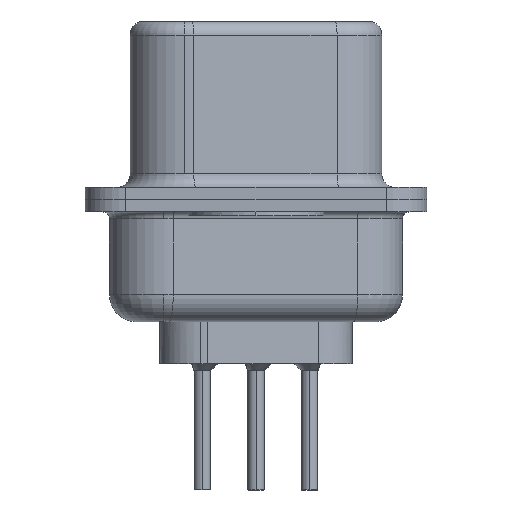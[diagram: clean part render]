
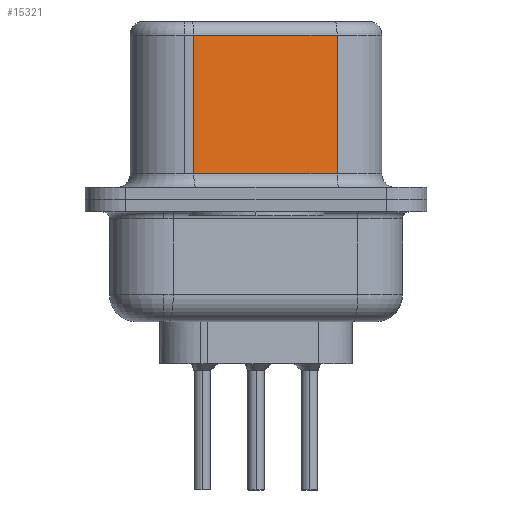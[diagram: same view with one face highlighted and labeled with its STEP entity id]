
A CAD part, left-side view. The second image highlights one B-rep face of the part: STEP entity #15321.
In plain terms, the highlighted planar face has unit normal (-0.985, -0.174, 0).
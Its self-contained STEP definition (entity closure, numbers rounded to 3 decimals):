
#120 = VECTOR ( 'NONE', #17267, 1000. ) ;
#445 = VECTOR ( 'NONE', #6712, 1000. ) ;
#1651 = FACE_OUTER_BOUND ( 'NONE', #18464, .T. ) ;
#1810 = ORIENTED_EDGE ( 'NONE', *, *, #16075, .T. ) ;
#2435 = DIRECTION ( 'NONE',  ( -0.174, 0.985, 0. ) ) ;
#2598 = ORIENTED_EDGE ( 'NONE', *, *, #7404, .T. ) ;
#3261 = CARTESIAN_POINT ( 'NONE',  ( 4.546, -2.987, 0.95 ) ) ;
#3389 = CARTESIAN_POINT ( 'NONE',  ( 4.546, -2.987, 6.07 ) ) ;
#5080 = CARTESIAN_POINT ( 'NONE',  ( 4.546, -2.987, 0.95 ) ) ;
#5292 = CARTESIAN_POINT ( 'NONE',  ( 3.615, 2.293, 6.57 ) ) ;
#5322 = DIRECTION ( 'NONE',  ( 0.985, 0.174, 0. ) ) ;
#6712 = DIRECTION ( 'NONE',  ( 0., 0., -1. ) ) ;
#7129 = VERTEX_POINT ( 'NONE', #10945 ) ;
#7404 = EDGE_CURVE ( 'NONE', #10019, #13987, #13589, .T. ) ;
#7949 = AXIS2_PLACEMENT_3D ( 'NONE', #15973, #5322, #2435 ) ;
#8676 = CARTESIAN_POINT ( 'NONE',  ( 3.615, 2.293, 6.07 ) ) ;
#8849 = EDGE_CURVE ( 'NONE', #7129, #10113, #10513, .T. ) ;
#9693 = LINE ( 'NONE', #3261, #11330 ) ;
#9973 = ORIENTED_EDGE ( 'NONE', *, *, #13278, .T. ) ;
#10019 = VERTEX_POINT ( 'NONE', #8676 ) ;
#10113 = VERTEX_POINT ( 'NONE', #5080 ) ;
#10513 = LINE ( 'NONE', #12588, #120 ) ;
#10945 = CARTESIAN_POINT ( 'NONE',  ( 4.546, -2.987, 6.07 ) ) ;
#11330 = VECTOR ( 'NONE', #16568, 1000. ) ;
#12588 = CARTESIAN_POINT ( 'NONE',  ( 4.546, -2.987, 6.57 ) ) ;
#13136 = PLANE ( 'NONE',  #7949 ) ;
#13278 = EDGE_CURVE ( 'NONE', #13987, #10113, #9693, .T. ) ;
#13427 = LINE ( 'NONE', #3389, #16704 ) ;
#13589 = LINE ( 'NONE', #5292, #445 ) ;
#13987 = VERTEX_POINT ( 'NONE', #17175 ) ;
#15321 = ADVANCED_FACE ( 'NONE', ( #1651 ), #13136, .F. ) ;
#15973 = CARTESIAN_POINT ( 'NONE',  ( 4.546, -2.987, 6.57 ) ) ;
#16075 = EDGE_CURVE ( 'NONE', #7129, #10019, #13427, .T. ) ;
#16568 = DIRECTION ( 'NONE',  ( 0.174, -0.985, 0. ) ) ;
#16704 = VECTOR ( 'NONE', #18339, 1000. ) ;
#17175 = CARTESIAN_POINT ( 'NONE',  ( 3.615, 2.293, 0.95 ) ) ;
#17267 = DIRECTION ( 'NONE',  ( 0., 0., -1. ) ) ;
#17385 = ORIENTED_EDGE ( 'NONE', *, *, #8849, .F. ) ;
#18339 = DIRECTION ( 'NONE',  ( -0.174, 0.985, 0. ) ) ;
#18464 = EDGE_LOOP ( 'NONE', ( #17385, #1810, #2598, #9973 ) ) ;
